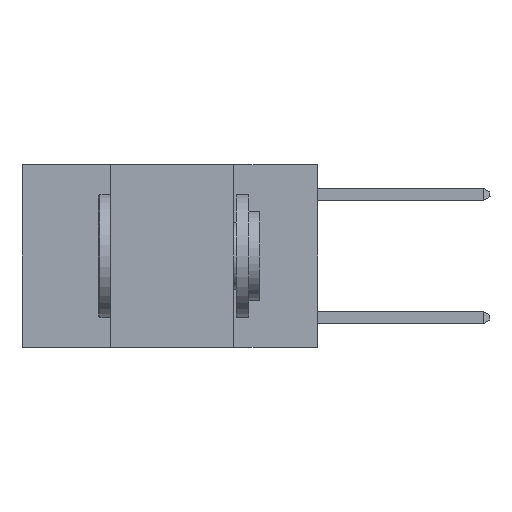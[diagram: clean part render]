
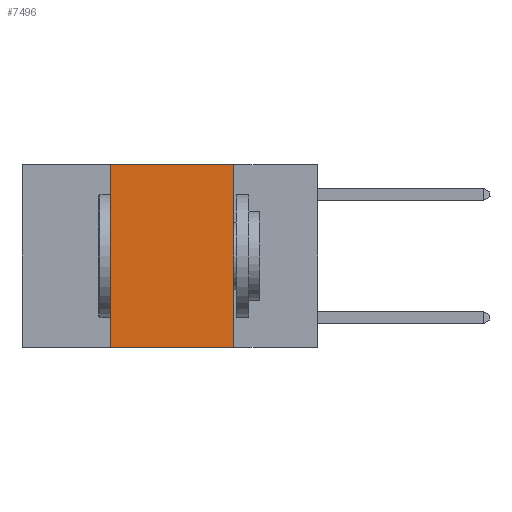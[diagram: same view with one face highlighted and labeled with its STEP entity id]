
A CAD part, left-side view. The second image highlights one B-rep face of the part: STEP entity #7496.
In plain terms, the highlighted planar face has unit normal (-1, 0, 0).
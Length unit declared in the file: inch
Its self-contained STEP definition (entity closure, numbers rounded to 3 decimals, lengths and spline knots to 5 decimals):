
#597 = DIRECTION ( 'NONE',  ( 1., 0., 0. ) ) ;
#625 = ORIENTED_EDGE ( 'NONE', *, *, #9253, .F. ) ;
#759 = DIRECTION ( 'NONE',  ( 0., 0., -1. ) ) ;
#1765 = VECTOR ( 'NONE', #15378, 39.37008 ) ;
#1837 = ORIENTED_EDGE ( 'NONE', *, *, #9344, .F. ) ;
#1904 = CARTESIAN_POINT ( 'NONE',  ( 0., 0.42, -0.37 ) ) ;
#2147 = VERTEX_POINT ( 'NONE', #7619 ) ;
#2696 = LINE ( 'NONE', #5339, #1765 ) ;
#2797 = VERTEX_POINT ( 'NONE', #6318 ) ;
#3017 = EDGE_LOOP ( 'NONE', ( #4615, #625, #1837, #11220 ) ) ;
#4486 = LINE ( 'NONE', #4654, #9291 ) ;
#4615 = ORIENTED_EDGE ( 'NONE', *, *, #5442, .F. ) ;
#4654 = CARTESIAN_POINT ( 'NONE',  ( 0., 0.42, 0. ) ) ;
#4741 = VECTOR ( 'NONE', #9866, 39.37008 ) ;
#5339 = CARTESIAN_POINT ( 'NONE',  ( 0., 0.17, 0. ) ) ;
#5442 = EDGE_CURVE ( 'NONE', #14158, #2797, #2696, .T. ) ;
#5703 = LINE ( 'NONE', #16139, #4741 ) ;
#5959 = DIRECTION ( 'NONE',  ( 0., 0., 1. ) ) ;
#6318 = CARTESIAN_POINT ( 'NONE',  ( 0., 0.17, -0.37 ) ) ;
#6586 = CARTESIAN_POINT ( 'NONE',  ( 0., 0.17, 0. ) ) ;
#6983 = AXIS2_PLACEMENT_3D ( 'NONE', #14730, #597, #759 ) ;
#7496 = ADVANCED_FACE ( 'NONE', ( #15779 ), #9755, .F. ) ;
#7619 = CARTESIAN_POINT ( 'NONE',  ( 0., 0.42, 0. ) ) ;
#9253 = EDGE_CURVE ( 'NONE', #2147, #14158, #14553, .T. ) ;
#9291 = VECTOR ( 'NONE', #5959, 39.37008 ) ;
#9341 = VERTEX_POINT ( 'NONE', #1904 ) ;
#9344 = EDGE_CURVE ( 'NONE', #9341, #2147, #4486, .T. ) ;
#9755 = PLANE ( 'NONE',  #6983 ) ;
#9866 = DIRECTION ( 'NONE',  ( 0., -1., 0. ) ) ;
#11220 = ORIENTED_EDGE ( 'NONE', *, *, #12563, .T. ) ;
#11633 = VECTOR ( 'NONE', #12014, 39.37008 ) ;
#12014 = DIRECTION ( 'NONE',  ( 0., -1., 0. ) ) ;
#12563 = EDGE_CURVE ( 'NONE', #9341, #2797, #5703, .T. ) ;
#14158 = VERTEX_POINT ( 'NONE', #6586 ) ;
#14385 = CARTESIAN_POINT ( 'NONE',  ( 0., 0.6, 0. ) ) ;
#14553 = LINE ( 'NONE', #14385, #11633 ) ;
#14730 = CARTESIAN_POINT ( 'NONE',  ( 0., 0.6, 0. ) ) ;
#15378 = DIRECTION ( 'NONE',  ( 0., 0., -1. ) ) ;
#15779 = FACE_OUTER_BOUND ( 'NONE', #3017, .T. ) ;
#16139 = CARTESIAN_POINT ( 'NONE',  ( 0., 0.6, -0.37 ) ) ;
